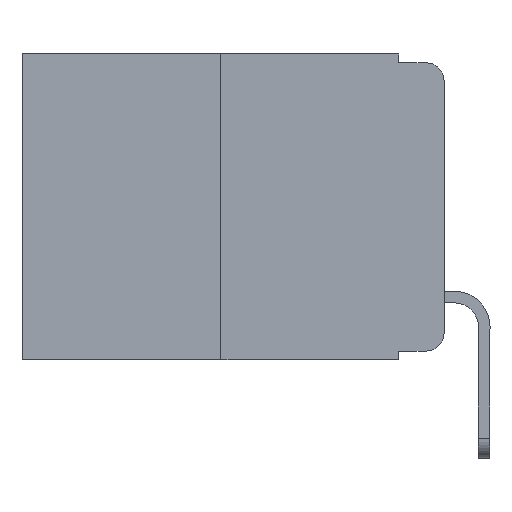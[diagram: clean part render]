
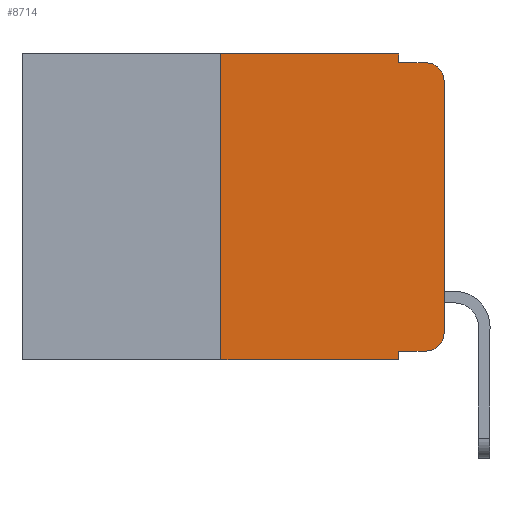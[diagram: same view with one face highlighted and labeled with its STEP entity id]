
A CAD part, left-side view. The second image highlights one B-rep face of the part: STEP entity #8714.
In plain terms, the highlighted planar face has unit normal (-1, 0, 0).
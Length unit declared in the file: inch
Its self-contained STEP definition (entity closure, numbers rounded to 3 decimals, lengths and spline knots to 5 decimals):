
#86 = VERTEX_POINT ( 'NONE', #14332 ) ;
#133 = LINE ( 'NONE', #5355, #16222 ) ;
#177 = CARTESIAN_POINT ( 'NONE',  ( 0., 0.051, -0.333 ) ) ;
#390 = DIRECTION ( 'NONE',  ( 0., 0., 1. ) ) ;
#713 = AXIS2_PLACEMENT_3D ( 'NONE', #15163, #6246, #16611 ) ;
#725 = VECTOR ( 'NONE', #14211, 39.37008 ) ;
#734 = CARTESIAN_POINT ( 'NONE',  ( 0., 0.02, -0.333 ) ) ;
#1971 = LINE ( 'NONE', #5625, #5496 ) ;
#2130 = ORIENTED_EDGE ( 'NONE', *, *, #9967, .F. ) ;
#3914 = CIRCLE ( 'NONE', #713, 0.02 ) ;
#4059 = CARTESIAN_POINT ( 'NONE',  ( 0., 0., -0.313 ) ) ;
#4346 = VECTOR ( 'NONE', #15652, 39.37008 ) ;
#4355 = PLANE ( 'NONE',  #4903 ) ;
#4651 = VECTOR ( 'NONE', #10652, 39.37008 ) ;
#4653 = ORIENTED_EDGE ( 'NONE', *, *, #9886, .T. ) ;
#4903 = AXIS2_PLACEMENT_3D ( 'NONE', #17461, #14834, #5874 ) ;
#4972 = CARTESIAN_POINT ( 'NONE',  ( 0., 0., -0.03 ) ) ;
#5147 = ORIENTED_EDGE ( 'NONE', *, *, #9919, .F. ) ;
#5355 = CARTESIAN_POINT ( 'NONE',  ( 0., 0.051, 0. ) ) ;
#5496 = VECTOR ( 'NONE', #17310, 39.37008 ) ;
#5536 = CARTESIAN_POINT ( 'NONE',  ( 0., 0.25, -0.343 ) ) ;
#5625 = CARTESIAN_POINT ( 'NONE',  ( 0., 0.473, -0.343 ) ) ;
#5874 = DIRECTION ( 'NONE',  ( 0., 0., -1. ) ) ;
#5912 = VERTEX_POINT ( 'NONE', #4059 ) ;
#5991 = VECTOR ( 'NONE', #18398, 39.37008 ) ;
#6091 = VERTEX_POINT ( 'NONE', #177 ) ;
#6246 = DIRECTION ( 'NONE',  ( -1., 0., 0. ) ) ;
#6623 = DIRECTION ( 'NONE',  ( -1., 0., 0. ) ) ;
#6980 = EDGE_CURVE ( 'NONE', #15955, #9442, #1971, .T. ) ;
#7095 = ORIENTED_EDGE ( 'NONE', *, *, #10030, .T. ) ;
#7238 = LINE ( 'NONE', #8168, #9913 ) ;
#7503 = VERTEX_POINT ( 'NONE', #18913 ) ;
#8168 = CARTESIAN_POINT ( 'NONE',  ( 0., 0., 0. ) ) ;
#8334 = EDGE_CURVE ( 'NONE', #11125, #86, #12802, .T. ) ;
#8714 = ADVANCED_FACE ( 'NONE', ( #15801 ), #4355, .F. ) ;
#8979 = LINE ( 'NONE', #14274, #4346 ) ;
#9418 = LINE ( 'NONE', #9838, #725 ) ;
#9442 = VERTEX_POINT ( 'NONE', #12785 ) ;
#9775 = ORIENTED_EDGE ( 'NONE', *, *, #9941, .F. ) ;
#9838 = CARTESIAN_POINT ( 'NONE',  ( 0., 0.051, 0. ) ) ;
#9884 = EDGE_CURVE ( 'NONE', #5912, #11613, #7238, .T. ) ;
#9886 = EDGE_CURVE ( 'NONE', #11613, #15375, #13753, .T. ) ;
#9913 = VECTOR ( 'NONE', #390, 39.37008 ) ;
#9919 = EDGE_CURVE ( 'NONE', #7503, #15375, #17040, .T. ) ;
#9941 = EDGE_CURVE ( 'NONE', #86, #7503, #9418, .T. ) ;
#9967 = EDGE_CURVE ( 'NONE', #15955, #11125, #8979, .T. ) ;
#9973 = EDGE_CURVE ( 'NONE', #6091, #9442, #133, .T. ) ;
#10030 = EDGE_CURVE ( 'NONE', #6091, #14567, #11108, .T. ) ;
#10345 = EDGE_CURVE ( 'NONE', #14567, #5912, #3914, .T. ) ;
#10652 = DIRECTION ( 'NONE',  ( 0., -1., 0. ) ) ;
#11108 = LINE ( 'NONE', #15910, #5991 ) ;
#11125 = VERTEX_POINT ( 'NONE', #18028 ) ;
#11234 = ORIENTED_EDGE ( 'NONE', *, *, #10345, .T. ) ;
#11613 = VERTEX_POINT ( 'NONE', #4972 ) ;
#11946 = CARTESIAN_POINT ( 'NONE',  ( 0., 0.02, -0.01 ) ) ;
#12280 = AXIS2_PLACEMENT_3D ( 'NONE', #15471, #6623, #16896 ) ;
#12370 = ORIENTED_EDGE ( 'NONE', *, *, #9884, .T. ) ;
#12785 = CARTESIAN_POINT ( 'NONE',  ( 0., 0.051, -0.343 ) ) ;
#12802 = LINE ( 'NONE', #18712, #4651 ) ;
#13261 = EDGE_LOOP ( 'NONE', ( #12370, #4653, #5147, #9775, #13640, #2130, #14081, #17661, #7095, #11234 ) ) ;
#13640 = ORIENTED_EDGE ( 'NONE', *, *, #8334, .F. ) ;
#13753 = CIRCLE ( 'NONE', #12280, 0.02 ) ;
#14081 = ORIENTED_EDGE ( 'NONE', *, *, #6980, .T. ) ;
#14141 = CARTESIAN_POINT ( 'NONE',  ( 0., 0.051, -0.01 ) ) ;
#14211 = DIRECTION ( 'NONE',  ( 0., 0., -1. ) ) ;
#14274 = CARTESIAN_POINT ( 'NONE',  ( 0., 0.25, 0. ) ) ;
#14332 = CARTESIAN_POINT ( 'NONE',  ( 0., 0.051, 0. ) ) ;
#14567 = VERTEX_POINT ( 'NONE', #734 ) ;
#14834 = DIRECTION ( 'NONE',  ( 1., 0., 0. ) ) ;
#15163 = CARTESIAN_POINT ( 'NONE',  ( 0., 0.02, -0.313 ) ) ;
#15375 = VERTEX_POINT ( 'NONE', #11946 ) ;
#15471 = CARTESIAN_POINT ( 'NONE',  ( 0., 0.02, -0.03 ) ) ;
#15652 = DIRECTION ( 'NONE',  ( 0., 0., 1. ) ) ;
#15721 = DIRECTION ( 'NONE',  ( 0., 0., -1. ) ) ;
#15801 = FACE_OUTER_BOUND ( 'NONE', #13261, .T. ) ;
#15910 = CARTESIAN_POINT ( 'NONE',  ( 0., 0.051, -0.333 ) ) ;
#15955 = VERTEX_POINT ( 'NONE', #5536 ) ;
#16222 = VECTOR ( 'NONE', #15721, 39.37008 ) ;
#16611 = DIRECTION ( 'NONE',  ( 0., 0., -1. ) ) ;
#16652 = VECTOR ( 'NONE', #18145, 39.37008 ) ;
#16896 = DIRECTION ( 'NONE',  ( 0., 0., -1. ) ) ;
#17040 = LINE ( 'NONE', #14141, #16652 ) ;
#17310 = DIRECTION ( 'NONE',  ( 0., -1., 0. ) ) ;
#17461 = CARTESIAN_POINT ( 'NONE',  ( 0., 0.473, 0. ) ) ;
#17661 = ORIENTED_EDGE ( 'NONE', *, *, #9973, .F. ) ;
#18028 = CARTESIAN_POINT ( 'NONE',  ( 0., 0.25, 0. ) ) ;
#18145 = DIRECTION ( 'NONE',  ( 0., -1., 0. ) ) ;
#18398 = DIRECTION ( 'NONE',  ( 0., -1., 0. ) ) ;
#18712 = CARTESIAN_POINT ( 'NONE',  ( 0., 0.473, 0. ) ) ;
#18913 = CARTESIAN_POINT ( 'NONE',  ( 0., 0.051, -0.01 ) ) ;
